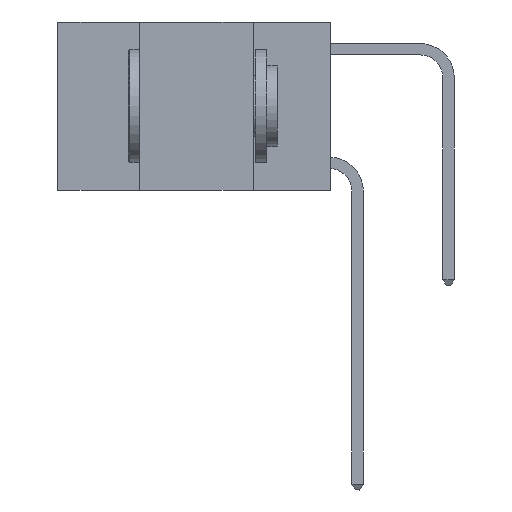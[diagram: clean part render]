
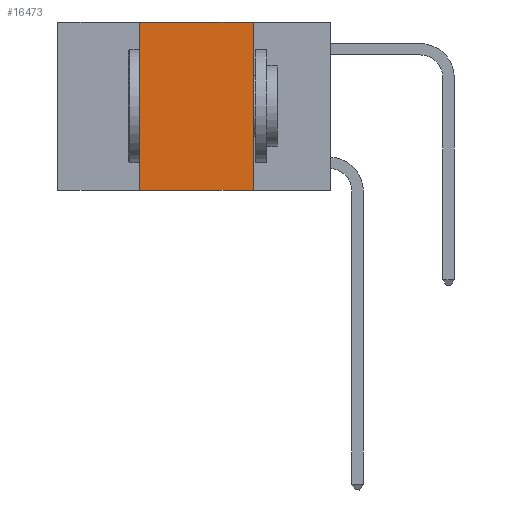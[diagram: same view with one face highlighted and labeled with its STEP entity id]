
A CAD part, left-side view. The second image highlights one B-rep face of the part: STEP entity #16473.
In plain terms, the highlighted planar face has unit normal (-1, 0, 0).
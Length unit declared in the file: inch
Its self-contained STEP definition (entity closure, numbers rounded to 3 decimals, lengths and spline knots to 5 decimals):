
#60 = VERTEX_POINT ( 'NONE', #18542 ) ;
#438 = DIRECTION ( 'NONE',  ( 0., -1., 0. ) ) ;
#1115 = EDGE_LOOP ( 'NONE', ( #2410, #5313, #1534, #1590 ) ) ;
#1534 = ORIENTED_EDGE ( 'NONE', *, *, #3564, .F. ) ;
#1590 = ORIENTED_EDGE ( 'NONE', *, *, #23846, .T. ) ;
#2410 = ORIENTED_EDGE ( 'NONE', *, *, #6697, .F. ) ;
#3518 = VECTOR ( 'NONE', #6951, 39.37008 ) ;
#3564 = EDGE_CURVE ( 'NONE', #25046, #60, #6225, .T. ) ;
#3615 = CARTESIAN_POINT ( 'NONE',  ( 0., 0.6, 0. ) ) ;
#4642 = CARTESIAN_POINT ( 'NONE',  ( 0., 0.42, -0.37 ) ) ;
#4792 = VECTOR ( 'NONE', #438, 39.37008 ) ;
#4798 = DIRECTION ( 'NONE',  ( 0., 0., -1. ) ) ;
#5313 = ORIENTED_EDGE ( 'NONE', *, *, #23780, .F. ) ;
#5642 = PLANE ( 'NONE',  #6832 ) ;
#6225 = LINE ( 'NONE', #18900, #22508 ) ;
#6697 = EDGE_CURVE ( 'NONE', #10230, #18136, #25469, .T. ) ;
#6832 = AXIS2_PLACEMENT_3D ( 'NONE', #3615, #11934, #14509 ) ;
#6951 = DIRECTION ( 'NONE',  ( 0., -1., 0. ) ) ;
#8262 = DIRECTION ( 'NONE',  ( 0., 0., 1. ) ) ;
#8310 = CARTESIAN_POINT ( 'NONE',  ( 0., 0.6, 0. ) ) ;
#10230 = VERTEX_POINT ( 'NONE', #17241 ) ;
#10515 = VECTOR ( 'NONE', #4798, 39.37008 ) ;
#11934 = DIRECTION ( 'NONE',  ( 1., 0., 0. ) ) ;
#12539 = LINE ( 'NONE', #8310, #4792 ) ;
#14509 = DIRECTION ( 'NONE',  ( 0., 0., -1. ) ) ;
#16473 = ADVANCED_FACE ( 'NONE', ( #24262 ), #5642, .F. ) ;
#17241 = CARTESIAN_POINT ( 'NONE',  ( 0., 0.17, 0. ) ) ;
#17364 = CARTESIAN_POINT ( 'NONE',  ( 0., 0.17, -0.37 ) ) ;
#18136 = VERTEX_POINT ( 'NONE', #17364 ) ;
#18542 = CARTESIAN_POINT ( 'NONE',  ( 0., 0.42, 0. ) ) ;
#18900 = CARTESIAN_POINT ( 'NONE',  ( 0., 0.42, 0. ) ) ;
#19212 = CARTESIAN_POINT ( 'NONE',  ( 0., 0.6, -0.37 ) ) ;
#22508 = VECTOR ( 'NONE', #8262, 39.37008 ) ;
#23424 = CARTESIAN_POINT ( 'NONE',  ( 0., 0.17, 0. ) ) ;
#23780 = EDGE_CURVE ( 'NONE', #60, #10230, #12539, .T. ) ;
#23795 = LINE ( 'NONE', #19212, #3518 ) ;
#23846 = EDGE_CURVE ( 'NONE', #25046, #18136, #23795, .T. ) ;
#24262 = FACE_OUTER_BOUND ( 'NONE', #1115, .T. ) ;
#25046 = VERTEX_POINT ( 'NONE', #4642 ) ;
#25469 = LINE ( 'NONE', #23424, #10515 ) ;
